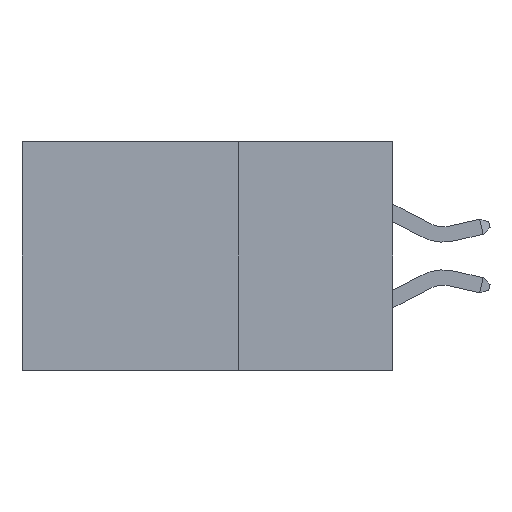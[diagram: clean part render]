
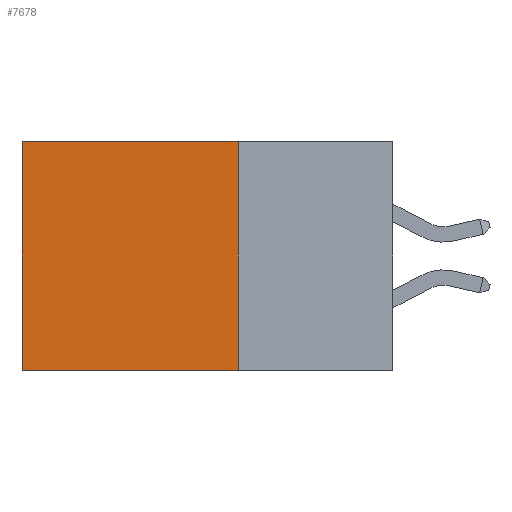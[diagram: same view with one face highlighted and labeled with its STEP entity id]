
A CAD part, left-side view. The second image highlights one B-rep face of the part: STEP entity #7678.
In plain terms, the highlighted planar face has unit normal (-1, 0, 0).
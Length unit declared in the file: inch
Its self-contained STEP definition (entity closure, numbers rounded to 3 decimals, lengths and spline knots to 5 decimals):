
#137 = DIRECTION ( 'NONE',  ( 0., 0., -1. ) ) ;
#231 = LINE ( 'NONE', #7627, #2450 ) ;
#345 = VERTEX_POINT ( 'NONE', #13001 ) ;
#606 = CARTESIAN_POINT ( 'NONE',  ( 0.2875, 0.6, 0. ) ) ;
#2114 = AXIS2_PLACEMENT_3D ( 'NONE', #10770, #13955, #10678 ) ;
#2285 = EDGE_CURVE ( 'NONE', #3907, #345, #10903, .T. ) ;
#2450 = VECTOR ( 'NONE', #12018, 39.37008 ) ;
#3771 = ORIENTED_EDGE ( 'NONE', *, *, #4224, .F. ) ;
#3818 = FACE_OUTER_BOUND ( 'NONE', #4436, .T. ) ;
#3865 = CARTESIAN_POINT ( 'NONE',  ( 0.2875, 0.25, 0. ) ) ;
#3907 = VERTEX_POINT ( 'NONE', #606 ) ;
#3997 = VECTOR ( 'NONE', #137, 39.37008 ) ;
#4224 = EDGE_CURVE ( 'NONE', #6543, #13526, #231, .T. ) ;
#4278 = DIRECTION ( 'NONE',  ( 0., 1., 0. ) ) ;
#4436 = EDGE_LOOP ( 'NONE', ( #13188, #8352, #3771, #5165 ) ) ;
#5165 = ORIENTED_EDGE ( 'NONE', *, *, #12891, .T. ) ;
#5482 = EDGE_CURVE ( 'NONE', #13526, #345, #6131, .T. ) ;
#5531 = CARTESIAN_POINT ( 'NONE',  ( 0.2875, 0.25, -0.37 ) ) ;
#6131 = LINE ( 'NONE', #5531, #11625 ) ;
#6252 = PLANE ( 'NONE',  #2114 ) ;
#6543 = VERTEX_POINT ( 'NONE', #3865 ) ;
#6899 = CARTESIAN_POINT ( 'NONE',  ( 0.2875, 0.25, -0.37 ) ) ;
#7627 = CARTESIAN_POINT ( 'NONE',  ( 0.2875, 0.25, 0. ) ) ;
#7678 = ADVANCED_FACE ( 'NONE', ( #3818 ), #6252, .F. ) ;
#7710 = CARTESIAN_POINT ( 'NONE',  ( 0.2875, 0.6, 0. ) ) ;
#8069 = VECTOR ( 'NONE', #12989, 39.37008 ) ;
#8352 = ORIENTED_EDGE ( 'NONE', *, *, #5482, .F. ) ;
#10678 = DIRECTION ( 'NONE',  ( 0., 0., -1. ) ) ;
#10770 = CARTESIAN_POINT ( 'NONE',  ( 0.2875, 0.25, 0. ) ) ;
#10903 = LINE ( 'NONE', #7710, #3997 ) ;
#11625 = VECTOR ( 'NONE', #4278, 39.37008 ) ;
#11699 = LINE ( 'NONE', #11861, #8069 ) ;
#11861 = CARTESIAN_POINT ( 'NONE',  ( 0.2875, 0.25, 0. ) ) ;
#12018 = DIRECTION ( 'NONE',  ( 0., 0., -1. ) ) ;
#12891 = EDGE_CURVE ( 'NONE', #6543, #3907, #11699, .T. ) ;
#12989 = DIRECTION ( 'NONE',  ( 0., 1., 0. ) ) ;
#13001 = CARTESIAN_POINT ( 'NONE',  ( 0.2875, 0.6, -0.37 ) ) ;
#13188 = ORIENTED_EDGE ( 'NONE', *, *, #2285, .T. ) ;
#13526 = VERTEX_POINT ( 'NONE', #6899 ) ;
#13955 = DIRECTION ( 'NONE',  ( 1., 0., 0. ) ) ;
